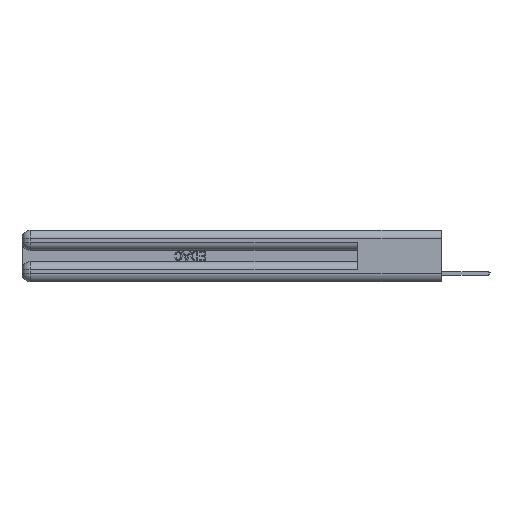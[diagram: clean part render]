
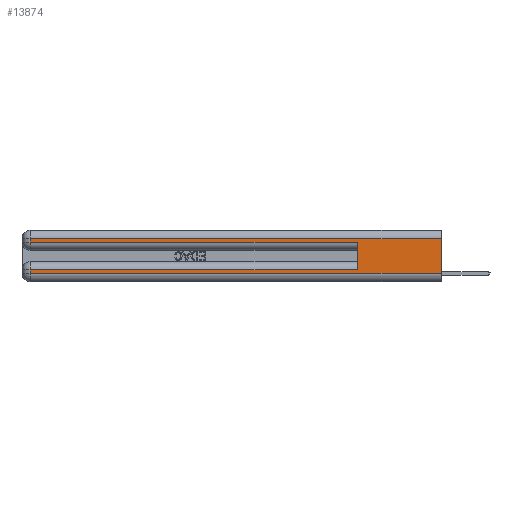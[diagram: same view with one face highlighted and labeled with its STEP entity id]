
A CAD part, left-side view. The second image highlights one B-rep face of the part: STEP entity #13874.
In plain terms, the highlighted planar face has unit normal (-1, 0, 0).
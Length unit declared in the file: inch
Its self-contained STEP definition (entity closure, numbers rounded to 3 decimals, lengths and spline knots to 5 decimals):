
#174 = VERTEX_POINT ( 'NONE', #3200 ) ;
#344 = DIRECTION ( 'NONE',  ( 0., 0., 1. ) ) ;
#559 = DIRECTION ( 'NONE',  ( 0., -1., 0. ) ) ;
#714 = DIRECTION ( 'NONE',  ( 1., 0., 0. ) ) ;
#1148 = LINE ( 'NONE', #23019, #20789 ) ;
#1423 = CARTESIAN_POINT ( 'NONE',  ( 0., 2.94, 0.085 ) ) ;
#1510 = VERTEX_POINT ( 'NONE', #27400 ) ;
#3016 = EDGE_CURVE ( 'NONE', #11109, #174, #19556, .T. ) ;
#3200 = CARTESIAN_POINT ( 'NONE',  ( 0., 2.94, 0.285 ) ) ;
#3374 = LINE ( 'NONE', #7570, #12573 ) ;
#4347 = DIRECTION ( 'NONE',  ( 0., 0., -1. ) ) ;
#4477 = VECTOR ( 'NONE', #13859, 39.37008 ) ;
#5372 = CARTESIAN_POINT ( 'NONE',  ( 0., 0., 0.31 ) ) ;
#7570 = CARTESIAN_POINT ( 'NONE',  ( 0., 2.94, 0.37 ) ) ;
#7626 = EDGE_CURVE ( 'NONE', #1510, #13191, #15357, .T. ) ;
#7775 = CARTESIAN_POINT ( 'NONE',  ( 0., 0., 0.285 ) ) ;
#8171 = CARTESIAN_POINT ( 'NONE',  ( 0., 2.94, 0.06 ) ) ;
#8616 = VECTOR ( 'NONE', #344, 39.37008 ) ;
#8968 = CARTESIAN_POINT ( 'NONE',  ( 0., 0., 0.06 ) ) ;
#8994 = EDGE_CURVE ( 'NONE', #1510, #11109, #11190, .T. ) ;
#9242 = EDGE_CURVE ( 'NONE', #15565, #13191, #14421, .T. ) ;
#11060 = VERTEX_POINT ( 'NONE', #22533 ) ;
#11109 = VERTEX_POINT ( 'NONE', #12752 ) ;
#11125 = CARTESIAN_POINT ( 'NONE',  ( 0., 0., 0.37 ) ) ;
#11174 = EDGE_CURVE ( 'NONE', #11060, #21383, #28337, .T. ) ;
#11190 = LINE ( 'NONE', #5372, #26862 ) ;
#11221 = CARTESIAN_POINT ( 'NONE',  ( 0., 0., 0.06 ) ) ;
#11523 = ORIENTED_EDGE ( 'NONE', *, *, #19060, .T. ) ;
#12573 = VECTOR ( 'NONE', #25434, 39.37008 ) ;
#12752 = CARTESIAN_POINT ( 'NONE',  ( 0., 2.94, 0.31 ) ) ;
#13031 = ORIENTED_EDGE ( 'NONE', *, *, #3016, .T. ) ;
#13191 = VERTEX_POINT ( 'NONE', #8968 ) ;
#13395 = ORIENTED_EDGE ( 'NONE', *, *, #11174, .F. ) ;
#13859 = DIRECTION ( 'NONE',  ( 0., 0., -1. ) ) ;
#13874 = ADVANCED_FACE ( 'NONE', ( #26677 ), #31554, .F. ) ;
#14269 = EDGE_CURVE ( 'NONE', #32890, #15565, #3374, .T. ) ;
#14421 = LINE ( 'NONE', #11221, #18024 ) ;
#15357 = LINE ( 'NONE', #11125, #4477 ) ;
#15530 = VECTOR ( 'NONE', #4347, 39.37008 ) ;
#15565 = VERTEX_POINT ( 'NONE', #8171 ) ;
#16037 = CARTESIAN_POINT ( 'NONE',  ( 0., 0., 0.37 ) ) ;
#17790 = ORIENTED_EDGE ( 'NONE', *, *, #9242, .T. ) ;
#18024 = VECTOR ( 'NONE', #18881, 39.37008 ) ;
#18249 = ORIENTED_EDGE ( 'NONE', *, *, #21624, .T. ) ;
#18615 = EDGE_LOOP ( 'NONE', ( #32603, #21888, #13031, #11523, #13395, #18249, #30868, #17790 ) ) ;
#18881 = DIRECTION ( 'NONE',  ( 0., -1., 0. ) ) ;
#19060 = EDGE_CURVE ( 'NONE', #174, #21383, #29025, .T. ) ;
#19160 = AXIS2_PLACEMENT_3D ( 'NONE', #16037, #714, #28743 ) ;
#19556 = LINE ( 'NONE', #22650, #15530 ) ;
#20207 = CARTESIAN_POINT ( 'NONE',  ( 0., 0.6, 0.285 ) ) ;
#20632 = DIRECTION ( 'NONE',  ( 0., 1., 0. ) ) ;
#20789 = VECTOR ( 'NONE', #20632, 39.37008 ) ;
#21383 = VERTEX_POINT ( 'NONE', #20207 ) ;
#21624 = EDGE_CURVE ( 'NONE', #11060, #32890, #1148, .T. ) ;
#21888 = ORIENTED_EDGE ( 'NONE', *, *, #8994, .T. ) ;
#22533 = CARTESIAN_POINT ( 'NONE',  ( 0., 0.6, 0.085 ) ) ;
#22650 = CARTESIAN_POINT ( 'NONE',  ( 0., 2.94, 0.37 ) ) ;
#23019 = CARTESIAN_POINT ( 'NONE',  ( 0., 0., 0.085 ) ) ;
#23417 = CARTESIAN_POINT ( 'NONE',  ( 0., 0.6, 0.145 ) ) ;
#24972 = VECTOR ( 'NONE', #559, 39.37008 ) ;
#25434 = DIRECTION ( 'NONE',  ( 0., 0., -1. ) ) ;
#26677 = FACE_OUTER_BOUND ( 'NONE', #18615, .T. ) ;
#26862 = VECTOR ( 'NONE', #28302, 39.37008 ) ;
#27400 = CARTESIAN_POINT ( 'NONE',  ( 0., 0., 0.31 ) ) ;
#28302 = DIRECTION ( 'NONE',  ( 0., 1., 0. ) ) ;
#28337 = LINE ( 'NONE', #23417, #8616 ) ;
#28743 = DIRECTION ( 'NONE',  ( 0., 0., -1. ) ) ;
#29025 = LINE ( 'NONE', #7775, #24972 ) ;
#30868 = ORIENTED_EDGE ( 'NONE', *, *, #14269, .T. ) ;
#31554 = PLANE ( 'NONE',  #19160 ) ;
#32603 = ORIENTED_EDGE ( 'NONE', *, *, #7626, .F. ) ;
#32890 = VERTEX_POINT ( 'NONE', #1423 ) ;
